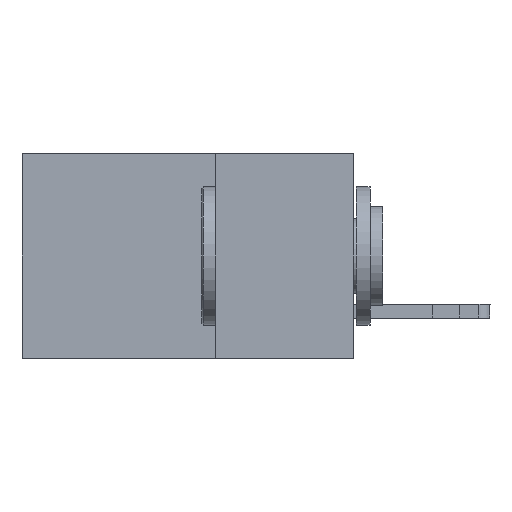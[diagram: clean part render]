
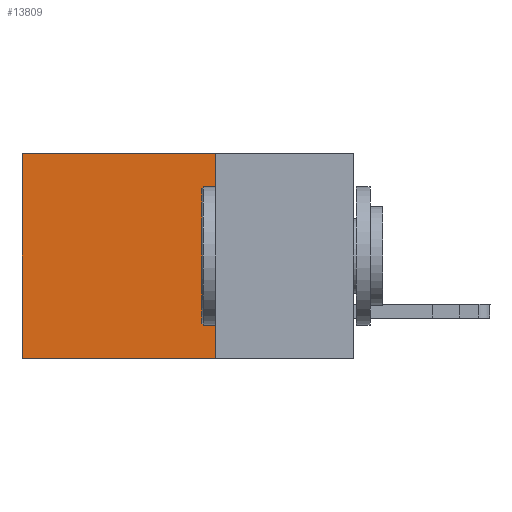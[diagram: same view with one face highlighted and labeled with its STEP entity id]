
A CAD part, left-side view. The second image highlights one B-rep face of the part: STEP entity #13809.
In plain terms, the highlighted planar face has unit normal (-1, 0, 0).
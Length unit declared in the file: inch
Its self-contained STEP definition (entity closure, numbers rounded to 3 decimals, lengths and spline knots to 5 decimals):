
#338 = LINE ( 'NONE', #9530, #3496 ) ;
#467 = VECTOR ( 'NONE', #16108, 39.37008 ) ;
#597 = VERTEX_POINT ( 'NONE', #10956 ) ;
#1212 = ORIENTED_EDGE ( 'NONE', *, *, #15415, .T. ) ;
#1291 = PLANE ( 'NONE',  #14970 ) ;
#2377 = LINE ( 'NONE', #17060, #5328 ) ;
#2547 = EDGE_CURVE ( 'NONE', #597, #14911, #16580, .T. ) ;
#3060 = DIRECTION ( 'NONE',  ( 0., 0., -1. ) ) ;
#3496 = VECTOR ( 'NONE', #9598, 39.37008 ) ;
#3830 = CARTESIAN_POINT ( 'NONE',  ( 0.2875, 0.6, -0.37 ) ) ;
#4051 = ORIENTED_EDGE ( 'NONE', *, *, #16570, .F. ) ;
#5328 = VECTOR ( 'NONE', #15792, 39.37008 ) ;
#6376 = ORIENTED_EDGE ( 'NONE', *, *, #7863, .F. ) ;
#6416 = CARTESIAN_POINT ( 'NONE',  ( 0.2875, 0.6, 0. ) ) ;
#7456 = EDGE_LOOP ( 'NONE', ( #11015, #6376, #4051, #1212 ) ) ;
#7666 = CARTESIAN_POINT ( 'NONE',  ( 0.2875, 0.25, 0. ) ) ;
#7863 = EDGE_CURVE ( 'NONE', #15181, #14911, #338, .T. ) ;
#9530 = CARTESIAN_POINT ( 'NONE',  ( 0.2875, 0.25, -0.37 ) ) ;
#9598 = DIRECTION ( 'NONE',  ( 0., 1., 0. ) ) ;
#10831 = DIRECTION ( 'NONE',  ( 1., 0., 0. ) ) ;
#10956 = CARTESIAN_POINT ( 'NONE',  ( 0.2875, 0.6, 0. ) ) ;
#11015 = ORIENTED_EDGE ( 'NONE', *, *, #2547, .T. ) ;
#11335 = DIRECTION ( 'NONE',  ( 0., 0., -1. ) ) ;
#11341 = LINE ( 'NONE', #12604, #14470 ) ;
#12604 = CARTESIAN_POINT ( 'NONE',  ( 0.2875, 0.25, 0. ) ) ;
#13292 = CARTESIAN_POINT ( 'NONE',  ( 0.2875, 0.25, 0. ) ) ;
#13809 = ADVANCED_FACE ( 'NONE', ( #14744 ), #1291, .F. ) ;
#14470 = VECTOR ( 'NONE', #11335, 39.37008 ) ;
#14744 = FACE_OUTER_BOUND ( 'NONE', #7456, .T. ) ;
#14911 = VERTEX_POINT ( 'NONE', #3830 ) ;
#14970 = AXIS2_PLACEMENT_3D ( 'NONE', #13292, #10831, #3060 ) ;
#15181 = VERTEX_POINT ( 'NONE', #16478 ) ;
#15415 = EDGE_CURVE ( 'NONE', #15918, #597, #2377, .T. ) ;
#15792 = DIRECTION ( 'NONE',  ( 0., 1., 0. ) ) ;
#15918 = VERTEX_POINT ( 'NONE', #7666 ) ;
#16108 = DIRECTION ( 'NONE',  ( 0., 0., -1. ) ) ;
#16478 = CARTESIAN_POINT ( 'NONE',  ( 0.2875, 0.25, -0.37 ) ) ;
#16570 = EDGE_CURVE ( 'NONE', #15918, #15181, #11341, .T. ) ;
#16580 = LINE ( 'NONE', #6416, #467 ) ;
#17060 = CARTESIAN_POINT ( 'NONE',  ( 0.2875, 0.25, 0. ) ) ;
